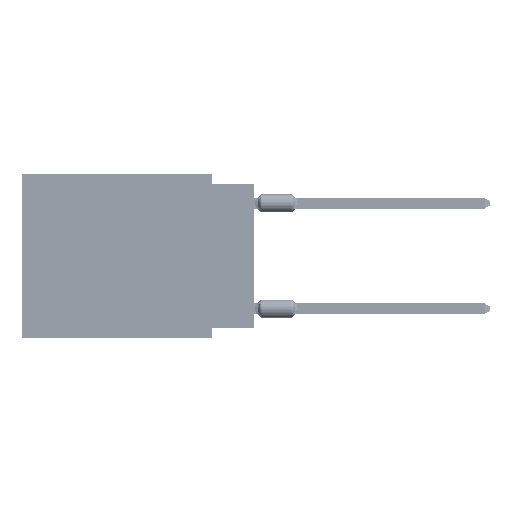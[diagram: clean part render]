
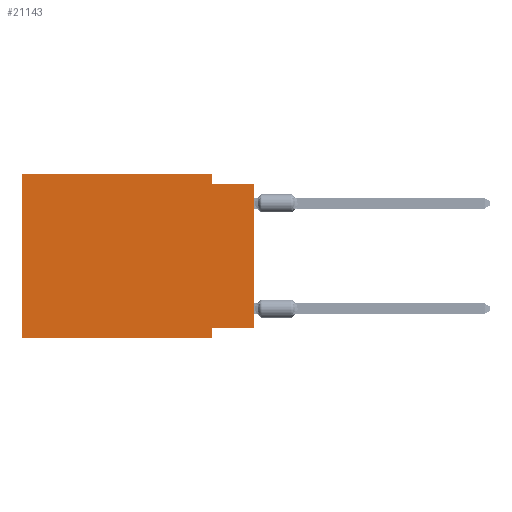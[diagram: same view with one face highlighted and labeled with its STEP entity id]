
A CAD part, left-side view. The second image highlights one B-rep face of the part: STEP entity #21143.
In plain terms, the highlighted planar face has unit normal (-1, 0, 0).
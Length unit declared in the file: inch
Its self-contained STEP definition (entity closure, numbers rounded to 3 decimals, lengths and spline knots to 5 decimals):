
#717 = CARTESIAN_POINT ( 'NONE',  ( 0., 0., -0.365 ) ) ;
#1409 = CARTESIAN_POINT ( 'NONE',  ( 0., 0., 0. ) ) ;
#1489 = DIRECTION ( 'NONE',  ( 0., -1., 0. ) ) ;
#3609 = EDGE_CURVE ( 'NONE', #58935, #67589, #43720, .T. ) ;
#7054 = CARTESIAN_POINT ( 'NONE',  ( 0., 0., -0.365 ) ) ;
#8205 = LINE ( 'NONE', #34712, #33089 ) ;
#9737 = EDGE_CURVE ( 'NONE', #60374, #32761, #39005, .T. ) ;
#10256 = LINE ( 'NONE', #83984, #58798 ) ;
#11025 = FACE_OUTER_BOUND ( 'NONE', #67223, .T. ) ;
#11297 = VERTEX_POINT ( 'NONE', #72052 ) ;
#15426 = ORIENTED_EDGE ( 'NONE', *, *, #17622, .F. ) ;
#17622 = EDGE_CURVE ( 'NONE', #68471, #60374, #59122, .T. ) ;
#19273 = ORIENTED_EDGE ( 'NONE', *, *, #3609, .F. ) ;
#19384 = EDGE_CURVE ( 'NONE', #67589, #83644, #8205, .T. ) ;
#21143 = ADVANCED_FACE ( 'NONE', ( #11025 ), #30895, .F. ) ;
#22394 = CARTESIAN_POINT ( 'NONE',  ( 0., 0.55, -0.39 ) ) ;
#23829 = DIRECTION ( 'NONE',  ( 0., 0., -1. ) ) ;
#24058 = CARTESIAN_POINT ( 'NONE',  ( 0., 0.1, 0. ) ) ;
#27453 = DIRECTION ( 'NONE',  ( 0., 0., 1. ) ) ;
#30389 = CARTESIAN_POINT ( 'NONE',  ( 0., 0.55, 0. ) ) ;
#30895 = PLANE ( 'NONE',  #67101 ) ;
#31516 = VECTOR ( 'NONE', #54545, 39.37008 ) ;
#31637 = CARTESIAN_POINT ( 'NONE',  ( 0., 0.1, -0.39 ) ) ;
#32761 = VERTEX_POINT ( 'NONE', #31637 ) ;
#33089 = VECTOR ( 'NONE', #54132, 39.37008 ) ;
#33628 = EDGE_CURVE ( 'NONE', #83644, #11297, #10256, .T. ) ;
#34712 = CARTESIAN_POINT ( 'NONE',  ( 0., 0.55, 0. ) ) ;
#35915 = CARTESIAN_POINT ( 'NONE',  ( 0., 0., -0.025 ) ) ;
#37523 = CARTESIAN_POINT ( 'NONE',  ( 0., 0.55, 0. ) ) ;
#39005 = LINE ( 'NONE', #71263, #69986 ) ;
#40754 = VERTEX_POINT ( 'NONE', #68005 ) ;
#41750 = LINE ( 'NONE', #73591, #58595 ) ;
#41994 = LINE ( 'NONE', #1409, #68779 ) ;
#42872 = EDGE_CURVE ( 'NONE', #58935, #32761, #41750, .T. ) ;
#43209 = CARTESIAN_POINT ( 'NONE',  ( 0., 0.1, -0.365 ) ) ;
#43480 = EDGE_CURVE ( 'NONE', #11297, #40754, #62384, .T. ) ;
#43720 = LINE ( 'NONE', #44157, #78882 ) ;
#44157 = CARTESIAN_POINT ( 'NONE',  ( 0., 0.55, 0. ) ) ;
#49983 = DIRECTION ( 'NONE',  ( 0., 0., -1. ) ) ;
#54129 = DIRECTION ( 'NONE',  ( 0., -1., 0. ) ) ;
#54132 = DIRECTION ( 'NONE',  ( 0., -1., 0. ) ) ;
#54545 = DIRECTION ( 'NONE',  ( 0., 1., 0. ) ) ;
#58595 = VECTOR ( 'NONE', #54129, 39.37008 ) ;
#58798 = VECTOR ( 'NONE', #49983, 39.37008 ) ;
#58935 = VERTEX_POINT ( 'NONE', #22394 ) ;
#59122 = LINE ( 'NONE', #717, #31516 ) ;
#59765 = EDGE_CURVE ( 'NONE', #68471, #40754, #41994, .T. ) ;
#60011 = VECTOR ( 'NONE', #1489, 39.37008 ) ;
#60374 = VERTEX_POINT ( 'NONE', #43209 ) ;
#62384 = LINE ( 'NONE', #35915, #60011 ) ;
#67101 = AXIS2_PLACEMENT_3D ( 'NONE', #37523, #79012, #23829 ) ;
#67223 = EDGE_LOOP ( 'NONE', ( #76801, #71869, #85140, #72513, #19273, #79690, #84571, #15426 ) ) ;
#67589 = VERTEX_POINT ( 'NONE', #30389 ) ;
#68005 = CARTESIAN_POINT ( 'NONE',  ( 0., 0., -0.025 ) ) ;
#68471 = VERTEX_POINT ( 'NONE', #7054 ) ;
#68779 = VECTOR ( 'NONE', #27453, 39.37008 ) ;
#69986 = VECTOR ( 'NONE', #85389, 39.37008 ) ;
#70223 = DIRECTION ( 'NONE',  ( 0., 0., 1. ) ) ;
#71263 = CARTESIAN_POINT ( 'NONE',  ( 0., 0.1, -0.39 ) ) ;
#71869 = ORIENTED_EDGE ( 'NONE', *, *, #43480, .F. ) ;
#72052 = CARTESIAN_POINT ( 'NONE',  ( 0., 0.1, -0.025 ) ) ;
#72513 = ORIENTED_EDGE ( 'NONE', *, *, #19384, .F. ) ;
#73591 = CARTESIAN_POINT ( 'NONE',  ( 0., 0.55, -0.39 ) ) ;
#76801 = ORIENTED_EDGE ( 'NONE', *, *, #59765, .T. ) ;
#78882 = VECTOR ( 'NONE', #70223, 39.37008 ) ;
#79012 = DIRECTION ( 'NONE',  ( 1., 0., 0. ) ) ;
#79690 = ORIENTED_EDGE ( 'NONE', *, *, #42872, .T. ) ;
#83644 = VERTEX_POINT ( 'NONE', #24058 ) ;
#83984 = CARTESIAN_POINT ( 'NONE',  ( 0., 0.1, 0. ) ) ;
#84571 = ORIENTED_EDGE ( 'NONE', *, *, #9737, .F. ) ;
#85140 = ORIENTED_EDGE ( 'NONE', *, *, #33628, .F. ) ;
#85389 = DIRECTION ( 'NONE',  ( 0., 0., -1. ) ) ;
